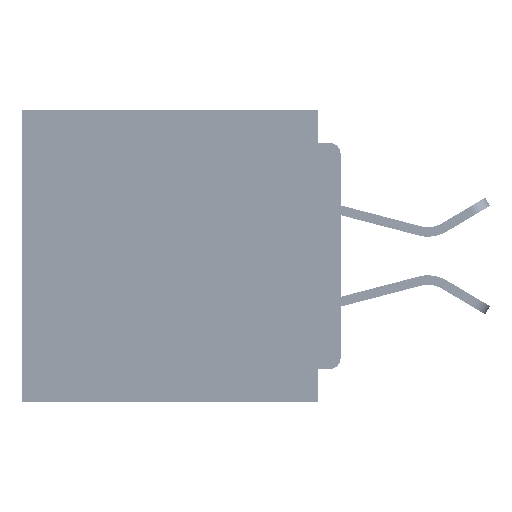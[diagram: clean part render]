
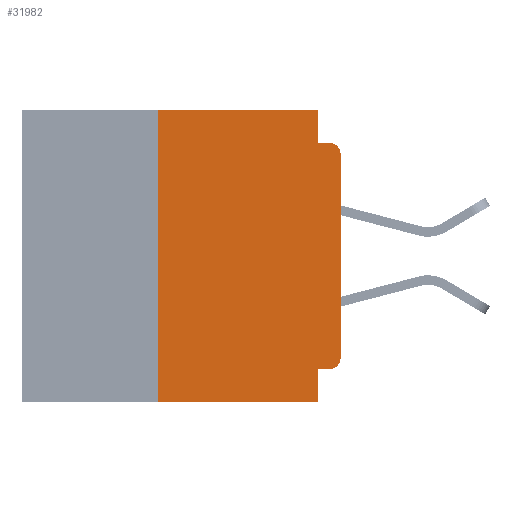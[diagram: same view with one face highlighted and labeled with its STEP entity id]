
A CAD part, left-side view. The second image highlights one B-rep face of the part: STEP entity #31982.
In plain terms, the highlighted planar face has unit normal (-1, 0, 0).
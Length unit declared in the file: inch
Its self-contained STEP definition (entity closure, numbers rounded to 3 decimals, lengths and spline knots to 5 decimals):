
#1805 = VERTEX_POINT ( 'NONE', #35776 ) ;
#2202 = CARTESIAN_POINT ( 'NONE',  ( 0., 0.25, -0.4 ) ) ;
#2263 = VECTOR ( 'NONE', #3242, 39.37008 ) ;
#2711 = EDGE_CURVE ( 'NONE', #62641, #69765, #51055, .T. ) ;
#3208 = ORIENTED_EDGE ( 'NONE', *, *, #17574, .F. ) ;
#3242 = DIRECTION ( 'NONE',  ( 0., -1., 0. ) ) ;
#3503 = PLANE ( 'NONE',  #20669 ) ;
#3726 = CARTESIAN_POINT ( 'NONE',  ( 0., 0.031, -0.4 ) ) ;
#4167 = FACE_OUTER_BOUND ( 'NONE', #58524, .T. ) ;
#5901 = CARTESIAN_POINT ( 'NONE',  ( 0., 0.437, -0.4 ) ) ;
#6033 = DIRECTION ( 'NONE',  ( 0., -1., 0. ) ) ;
#7689 = ORIENTED_EDGE ( 'NONE', *, *, #67885, .F. ) ;
#7873 = VECTOR ( 'NONE', #6033, 39.37008 ) ;
#8550 = CARTESIAN_POINT ( 'NONE',  ( 0., 0., 0. ) ) ;
#8825 = EDGE_CURVE ( 'NONE', #33604, #52360, #43574, .T. ) ;
#10131 = CARTESIAN_POINT ( 'NONE',  ( 0., 0.031, -0.4 ) ) ;
#10271 = EDGE_CURVE ( 'NONE', #64615, #28794, #58550, .T. ) ;
#11237 = CARTESIAN_POINT ( 'NONE',  ( 0., 0., -0.355 ) ) ;
#12768 = DIRECTION ( 'NONE',  ( 0., 0., 1. ) ) ;
#14798 = VECTOR ( 'NONE', #38252, 39.37008 ) ;
#15604 = DIRECTION ( 'NONE',  ( 0., 0., -1. ) ) ;
#16655 = ORIENTED_EDGE ( 'NONE', *, *, #35680, .F. ) ;
#17574 = EDGE_CURVE ( 'NONE', #28794, #33062, #22280, .T. ) ;
#19708 = CARTESIAN_POINT ( 'NONE',  ( 0., 0., -0.045 ) ) ;
#19845 = DIRECTION ( 'NONE',  ( 0., 0., -1. ) ) ;
#20669 = AXIS2_PLACEMENT_3D ( 'NONE', #68200, #52235, #19845 ) ;
#20676 = VECTOR ( 'NONE', #24923, 39.37008 ) ;
#21333 = CARTESIAN_POINT ( 'NONE',  ( 0., 0.015, -0.34 ) ) ;
#21559 = DIRECTION ( 'NONE',  ( -1., 0., 0. ) ) ;
#22084 = ORIENTED_EDGE ( 'NONE', *, *, #23742, .F. ) ;
#22280 = LINE ( 'NONE', #19708, #49333 ) ;
#22418 = VECTOR ( 'NONE', #12768, 39.37008 ) ;
#23742 = EDGE_CURVE ( 'NONE', #62641, #46606, #36785, .T. ) ;
#24923 = DIRECTION ( 'NONE',  ( 0., 0., 1. ) ) ;
#26168 = CARTESIAN_POINT ( 'NONE',  ( 0., 0.031, -0.355 ) ) ;
#26570 = CARTESIAN_POINT ( 'NONE',  ( 0., 0.25, 0. ) ) ;
#26810 = DIRECTION ( 'NONE',  ( 0., 0., -1. ) ) ;
#28569 = CARTESIAN_POINT ( 'NONE',  ( 0., 0.015, -0.045 ) ) ;
#28794 = VERTEX_POINT ( 'NONE', #56375 ) ;
#31982 = ADVANCED_FACE ( 'NONE', ( #4167 ), #3503, .F. ) ;
#32845 = ORIENTED_EDGE ( 'NONE', *, *, #34103, .T. ) ;
#33062 = VERTEX_POINT ( 'NONE', #28569 ) ;
#33604 = VERTEX_POINT ( 'NONE', #38439 ) ;
#34103 = EDGE_CURVE ( 'NONE', #33604, #1805, #45339, .T. ) ;
#34460 = LINE ( 'NONE', #46292, #2263 ) ;
#34740 = VERTEX_POINT ( 'NONE', #53630 ) ;
#34806 = ORIENTED_EDGE ( 'NONE', *, *, #51325, .T. ) ;
#35046 = LINE ( 'NONE', #8550, #20676 ) ;
#35680 = EDGE_CURVE ( 'NONE', #52360, #69765, #68785, .T. ) ;
#35776 = CARTESIAN_POINT ( 'NONE',  ( 0., 0., -0.34 ) ) ;
#36785 = LINE ( 'NONE', #61264, #22418 ) ;
#38252 = DIRECTION ( 'NONE',  ( 0., 1., 0. ) ) ;
#38439 = CARTESIAN_POINT ( 'NONE',  ( 0., 0.015, -0.355 ) ) ;
#41877 = DIRECTION ( 'NONE',  ( 0., 0., -1. ) ) ;
#43421 = EDGE_CURVE ( 'NONE', #1805, #34740, #35046, .T. ) ;
#43574 = LINE ( 'NONE', #11237, #14798 ) ;
#44179 = VECTOR ( 'NONE', #41877, 39.37008 ) ;
#45339 = CIRCLE ( 'NONE', #51096, 0.015 ) ;
#46292 = CARTESIAN_POINT ( 'NONE',  ( 0., 0.437, 0. ) ) ;
#46606 = VERTEX_POINT ( 'NONE', #26570 ) ;
#49333 = VECTOR ( 'NONE', #57524, 39.37008 ) ;
#50334 = ORIENTED_EDGE ( 'NONE', *, *, #2711, .T. ) ;
#51055 = LINE ( 'NONE', #5901, #7873 ) ;
#51096 = AXIS2_PLACEMENT_3D ( 'NONE', #21333, #59145, #26810 ) ;
#51325 = EDGE_CURVE ( 'NONE', #34740, #33062, #54101, .T. ) ;
#52235 = DIRECTION ( 'NONE',  ( 1., 0., 0. ) ) ;
#52360 = VERTEX_POINT ( 'NONE', #26168 ) ;
#52444 = ORIENTED_EDGE ( 'NONE', *, *, #10271, .F. ) ;
#53630 = CARTESIAN_POINT ( 'NONE',  ( 0., 0., -0.06 ) ) ;
#53929 = CARTESIAN_POINT ( 'NONE',  ( 0., 0.015, -0.06 ) ) ;
#54101 = CIRCLE ( 'NONE', #69193, 0.015 ) ;
#56375 = CARTESIAN_POINT ( 'NONE',  ( 0., 0.031, -0.045 ) ) ;
#57524 = DIRECTION ( 'NONE',  ( 0., -1., 0. ) ) ;
#57941 = CARTESIAN_POINT ( 'NONE',  ( 0., 0.031, 0. ) ) ;
#58524 = EDGE_LOOP ( 'NONE', ( #68154, #34806, #3208, #52444, #7689, #22084, #50334, #16655, #59897, #32845 ) ) ;
#58550 = LINE ( 'NONE', #57941, #44179 ) ;
#59145 = DIRECTION ( 'NONE',  ( -1., 0., 0. ) ) ;
#59348 = DIRECTION ( 'NONE',  ( 0., 0., -1. ) ) ;
#59897 = ORIENTED_EDGE ( 'NONE', *, *, #8825, .F. ) ;
#61264 = CARTESIAN_POINT ( 'NONE',  ( 0., 0.25, -0.4 ) ) ;
#62641 = VERTEX_POINT ( 'NONE', #2202 ) ;
#64615 = VERTEX_POINT ( 'NONE', #66708 ) ;
#66708 = CARTESIAN_POINT ( 'NONE',  ( 0., 0.031, 0. ) ) ;
#67110 = VECTOR ( 'NONE', #15604, 39.37008 ) ;
#67885 = EDGE_CURVE ( 'NONE', #46606, #64615, #34460, .T. ) ;
#68154 = ORIENTED_EDGE ( 'NONE', *, *, #43421, .T. ) ;
#68200 = CARTESIAN_POINT ( 'NONE',  ( 0., 0.437, 0. ) ) ;
#68785 = LINE ( 'NONE', #10131, #67110 ) ;
#69193 = AXIS2_PLACEMENT_3D ( 'NONE', #53929, #21559, #59348 ) ;
#69765 = VERTEX_POINT ( 'NONE', #3726 ) ;
